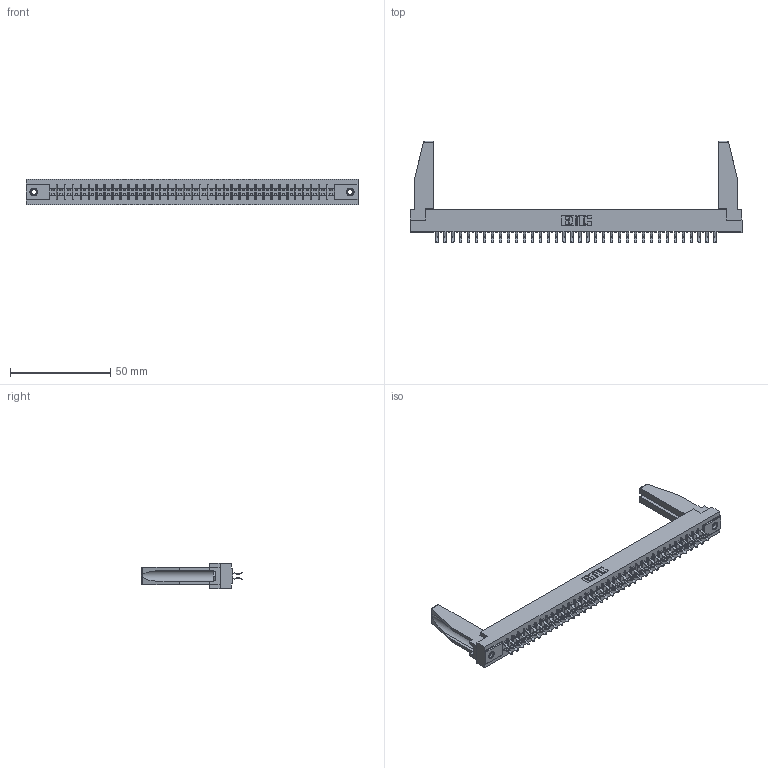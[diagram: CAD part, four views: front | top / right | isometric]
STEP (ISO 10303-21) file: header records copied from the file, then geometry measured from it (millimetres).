
FILE_DESCRIPTION (( 'STEP AP203' ), '1' );
FILE_NAME ('355-072-556-578.STEP', '2019-09-13T12:25:55', ( '' ), ( '' ), 'SwSTEP 2.0', 'SolidWorks 2016', '' );
FILE_SCHEMA (( 'CONFIG_CONTROL_DESIGN' ));
Length unit declared in the file: inch
Products named in the file (5): 345-250-001_345-250-001-102; 305-290-001_556; 355-072-556-578; 305 Part_.156 Dia; 307-220-078
Assembly tree (77 placements, depth 2):
  355-072-556-578
    305 Part_.156 Dia
    305-290-001_556  x72
    345-250-001_345-250-001-102  x2
    307-220-078  x2
Bounding box: 165.66 x 50.67 x 12.7 mm (x, y, z)
Volume: 20730.7 mm3; surface area: 25804.2 mm2
Topology: 77 solids, 77 shells, 4278 faces, 12274 edges, 7980 vertices
Faces by surface type: plane 2384, cylinder 1734, sphere 144, cone 12, torus 4
Entity records: 42370 total; most frequent: CARTESIAN_POINT 7020, ORIENTED_EDGE 6926, DIRECTION 6757, EDGE_CURVE 3463, VECTOR 2787, LINE 2787, VERTEX_POINT 2206, AXIS2_PLACEMENT_3D 1985
